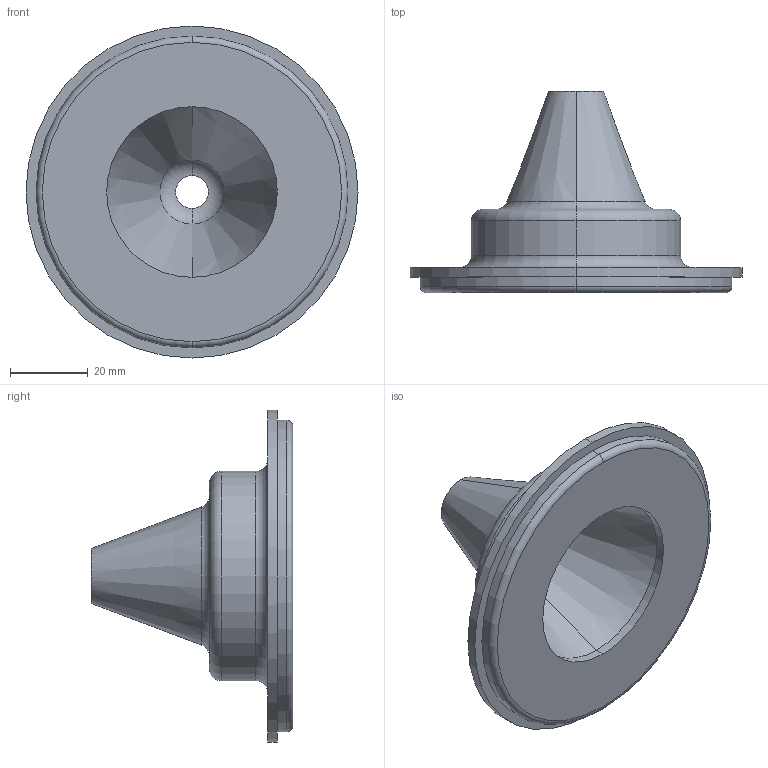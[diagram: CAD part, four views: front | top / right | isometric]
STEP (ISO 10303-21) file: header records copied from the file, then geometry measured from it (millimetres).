
FILE_DESCRIPTION (( 'STEP AP214' ), '1' );
FILE_NAME ('Rear_cover_02.STEP', '2024-01-26T08:57:26', ( '' ), ( '' ), 'SwSTEP 2.0', 'SolidWorks 2021', '' );
FILE_SCHEMA (( 'AUTOMOTIVE_DESIGN' ));
Length unit declared in the file: millimetre
Products named in the file (1): Rear_cover_02
Bounding box: 85.6 x 52 x 85.6 mm (x, y, z)
Volume: 53050.2 mm3; surface area: 19712.7 mm2
Topology: 1 solids, 1 shells, 31 faces, 62 edges, 36 vertices
Faces by surface type: torus 12, cylinder 10, plane 5, cone 4
Entity records: 854 total; most frequent: DIRECTION 174, CARTESIAN_POINT 130, ORIENTED_EDGE 124, AXIS2_PLACEMENT_3D 80, EDGE_CURVE 62, CIRCLE 48, VERTEX_POINT 36, EDGE_LOOP 36
